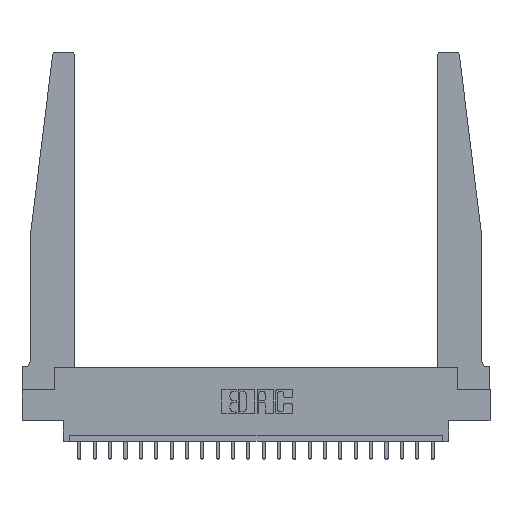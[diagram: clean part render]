
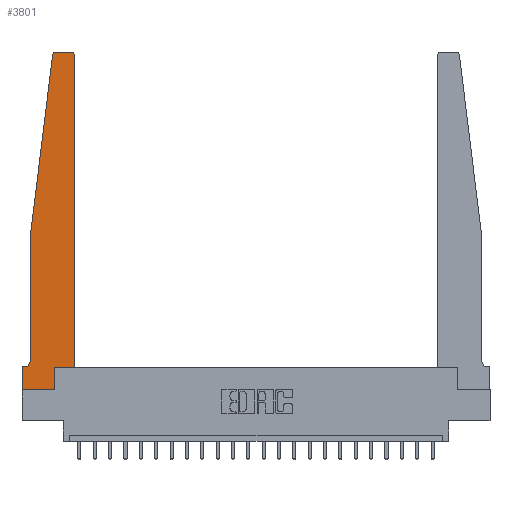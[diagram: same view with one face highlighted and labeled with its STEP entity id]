
A CAD part, top view. The second image highlights one B-rep face of the part: STEP entity #3801.
In plain terms, the highlighted planar face has unit normal (0, 0, 1).
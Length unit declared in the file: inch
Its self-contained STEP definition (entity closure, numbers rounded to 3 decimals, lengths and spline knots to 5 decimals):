
#557 = CIRCLE ( 'NONE', #19562, 0.03 ) ;
#636 = CARTESIAN_POINT ( 'NONE',  ( 0.395, 2.72, 0.37 ) ) ;
#779 = LINE ( 'NONE', #4105, #10875 ) ;
#983 = EDGE_LOOP ( 'NONE', ( #12375, #7026, #19817, #9304, #18638, #13432, #8237, #18020, #7289, #5497, #2859, #11993 ) ) ;
#1055 = CARTESIAN_POINT ( 'NONE',  ( 0.24675, 2.72367, 0.37 ) ) ;
#1247 = LINE ( 'NONE', #4476, #17745 ) ;
#1261 = CARTESIAN_POINT ( 'NONE',  ( 0.2605, 0.18, 0.37 ) ) ;
#1734 = EDGE_CURVE ( 'NONE', #5350, #15551, #1247, .T. ) ;
#1905 = LINE ( 'NONE', #13924, #12694 ) ;
#2113 = EDGE_CURVE ( 'NONE', #21769, #18946, #779, .T. ) ;
#2414 = LINE ( 'NONE', #19719, #10950 ) ;
#2510 = VECTOR ( 'NONE', #15008, 39.37008 ) ;
#2758 = LINE ( 'NONE', #14674, #2510 ) ;
#2859 = ORIENTED_EDGE ( 'NONE', *, *, #1734, .T. ) ;
#2923 = CARTESIAN_POINT ( 'NONE',  ( 0.25, 2.75, 0.37 ) ) ;
#3801 = ADVANCED_FACE ( 'NONE', ( #16862 ), #16748, .T. ) ;
#4105 = CARTESIAN_POINT ( 'NONE',  ( 0., 0., 0.37 ) ) ;
#4197 = DIRECTION ( 'NONE',  ( 0., 0., 1. ) ) ;
#4233 = EDGE_CURVE ( 'NONE', #21442, #8539, #21183, .T. ) ;
#4278 = CARTESIAN_POINT ( 'NONE',  ( 0.015, 0.2375, 0.37 ) ) ;
#4476 = CARTESIAN_POINT ( 'NONE',  ( 0.425, 0.18, 0.37 ) ) ;
#4506 = DIRECTION ( 'NONE',  ( -1., 0., 0. ) ) ;
#4529 = VERTEX_POINT ( 'NONE', #18070 ) ;
#5026 = AXIS2_PLACEMENT_3D ( 'NONE', #4278, #11271, #4506 ) ;
#5350 = VERTEX_POINT ( 'NONE', #6669 ) ;
#5497 = ORIENTED_EDGE ( 'NONE', *, *, #18047, .T. ) ;
#5527 = CARTESIAN_POINT ( 'NONE',  ( 0.27653, 2.75, 0.37 ) ) ;
#6161 = CARTESIAN_POINT ( 'NONE',  ( 0., 0., 0.37 ) ) ;
#6624 = CARTESIAN_POINT ( 'NONE',  ( 0.015, 0.1875, 0.37 ) ) ;
#6669 = CARTESIAN_POINT ( 'NONE',  ( 0.425, 0.18, 0.37 ) ) ;
#7026 = ORIENTED_EDGE ( 'NONE', *, *, #9834, .T. ) ;
#7260 = VECTOR ( 'NONE', #11290, 39.37008 ) ;
#7289 = ORIENTED_EDGE ( 'NONE', *, *, #22165, .T. ) ;
#7498 = DIRECTION ( 'NONE',  ( 1., 0., 0. ) ) ;
#7855 = CARTESIAN_POINT ( 'NONE',  ( 0.065, 0.2375, 0.37 ) ) ;
#7973 = LINE ( 'NONE', #2923, #8641 ) ;
#7995 = AXIS2_PLACEMENT_3D ( 'NONE', #20340, #8197, #16631 ) ;
#8008 = VERTEX_POINT ( 'NONE', #5527 ) ;
#8069 = EDGE_CURVE ( 'NONE', #4529, #21442, #2414, .T. ) ;
#8098 = EDGE_CURVE ( 'NONE', #18946, #17336, #2758, .T. ) ;
#8197 = DIRECTION ( 'NONE',  ( 0., 0., 1. ) ) ;
#8237 = ORIENTED_EDGE ( 'NONE', *, *, #2113, .T. ) ;
#8539 = VERTEX_POINT ( 'NONE', #6624 ) ;
#8641 = VECTOR ( 'NONE', #9922, 39.37008 ) ;
#9304 = ORIENTED_EDGE ( 'NONE', *, *, #8069, .T. ) ;
#9505 = DIRECTION ( 'NONE',  ( 0., -1., 0. ) ) ;
#9595 = DIRECTION ( 'NONE',  ( 1., 0., 0. ) ) ;
#9753 = CARTESIAN_POINT ( 'NONE',  ( 0.425, 2.72, 0.37 ) ) ;
#9834 = EDGE_CURVE ( 'NONE', #8008, #15116, #19888, .T. ) ;
#9922 = DIRECTION ( 'NONE',  ( -1., 0., 0. ) ) ;
#10629 = EDGE_CURVE ( 'NONE', #15116, #4529, #18426, .T. ) ;
#10875 = VECTOR ( 'NONE', #9505, 39.37008 ) ;
#10950 = VECTOR ( 'NONE', #16360, 39.37008 ) ;
#11024 = CARTESIAN_POINT ( 'NONE',  ( 0.065, 1.25, 0.37 ) ) ;
#11058 = LINE ( 'NONE', #20220, #7260 ) ;
#11271 = DIRECTION ( 'NONE',  ( 0., 0., -1. ) ) ;
#11290 = DIRECTION ( 'NONE',  ( -1., 0., 0. ) ) ;
#11477 = DIRECTION ( 'NONE',  ( 0., 1., 0. ) ) ;
#11907 = VERTEX_POINT ( 'NONE', #1261 ) ;
#11993 = ORIENTED_EDGE ( 'NONE', *, *, #20381, .T. ) ;
#12375 = ORIENTED_EDGE ( 'NONE', *, *, #21542, .T. ) ;
#12694 = VECTOR ( 'NONE', #20933, 39.37008 ) ;
#13432 = ORIENTED_EDGE ( 'NONE', *, *, #13696, .T. ) ;
#13696 = EDGE_CURVE ( 'NONE', #8539, #21769, #11058, .T. ) ;
#13924 = CARTESIAN_POINT ( 'NONE',  ( 0.2605, 0.18, 0.37 ) ) ;
#14336 = VERTEX_POINT ( 'NONE', #21215 ) ;
#14674 = CARTESIAN_POINT ( 'NONE',  ( 0., 0., 0.37 ) ) ;
#15008 = DIRECTION ( 'NONE',  ( 1., 0., 0. ) ) ;
#15116 = VERTEX_POINT ( 'NONE', #1055 ) ;
#15551 = VERTEX_POINT ( 'NONE', #9753 ) ;
#16231 = VECTOR ( 'NONE', #7498, 39.37008 ) ;
#16360 = DIRECTION ( 'NONE',  ( 0., -1., 0. ) ) ;
#16411 = DIRECTION ( 'NONE',  ( 1., 0., 0. ) ) ;
#16578 = DIRECTION ( 'NONE',  ( -0.122, -0.992, 0. ) ) ;
#16631 = DIRECTION ( 'NONE',  ( 1., 0., 0. ) ) ;
#16748 = PLANE ( 'NONE',  #7995 ) ;
#16862 = FACE_OUTER_BOUND ( 'NONE', #983, .T. ) ;
#17336 = VERTEX_POINT ( 'NONE', #18307 ) ;
#17745 = VECTOR ( 'NONE', #11477, 39.37008 ) ;
#17793 = CARTESIAN_POINT ( 'NONE',  ( 0.425, 0.18, 0.37 ) ) ;
#18020 = ORIENTED_EDGE ( 'NONE', *, *, #8098, .T. ) ;
#18047 = EDGE_CURVE ( 'NONE', #11907, #5350, #22417, .T. ) ;
#18070 = CARTESIAN_POINT ( 'NONE',  ( 0.065, 1.25, 0.37 ) ) ;
#18307 = CARTESIAN_POINT ( 'NONE',  ( 0.2605, 0., 0.37 ) ) ;
#18426 = LINE ( 'NONE', #11024, #22594 ) ;
#18638 = ORIENTED_EDGE ( 'NONE', *, *, #4233, .T. ) ;
#18946 = VERTEX_POINT ( 'NONE', #6161 ) ;
#19505 = AXIS2_PLACEMENT_3D ( 'NONE', #21629, #4197, #9595 ) ;
#19562 = AXIS2_PLACEMENT_3D ( 'NONE', #636, #21286, #16411 ) ;
#19719 = CARTESIAN_POINT ( 'NONE',  ( 0.065, 1.25, 0.37 ) ) ;
#19817 = ORIENTED_EDGE ( 'NONE', *, *, #10629, .T. ) ;
#19888 = CIRCLE ( 'NONE', #19505, 0.03 ) ;
#20220 = CARTESIAN_POINT ( 'NONE',  ( 0.065, 0.1875, 0.37 ) ) ;
#20340 = CARTESIAN_POINT ( 'NONE',  ( 0., 0.1875, 0.37 ) ) ;
#20381 = EDGE_CURVE ( 'NONE', #15551, #14336, #557, .T. ) ;
#20933 = DIRECTION ( 'NONE',  ( 0., 1., 0. ) ) ;
#21183 = CIRCLE ( 'NONE', #5026, 0.05 ) ;
#21215 = CARTESIAN_POINT ( 'NONE',  ( 0.395, 2.75, 0.37 ) ) ;
#21286 = DIRECTION ( 'NONE',  ( 0., 0., 1. ) ) ;
#21442 = VERTEX_POINT ( 'NONE', #7855 ) ;
#21542 = EDGE_CURVE ( 'NONE', #14336, #8008, #7973, .T. ) ;
#21629 = CARTESIAN_POINT ( 'NONE',  ( 0.27653, 2.72, 0.37 ) ) ;
#21769 = VERTEX_POINT ( 'NONE', #21931 ) ;
#21931 = CARTESIAN_POINT ( 'NONE',  ( 0., 0.1875, 0.37 ) ) ;
#22165 = EDGE_CURVE ( 'NONE', #17336, #11907, #1905, .T. ) ;
#22417 = LINE ( 'NONE', #17793, #16231 ) ;
#22594 = VECTOR ( 'NONE', #16578, 39.37008 ) ;
